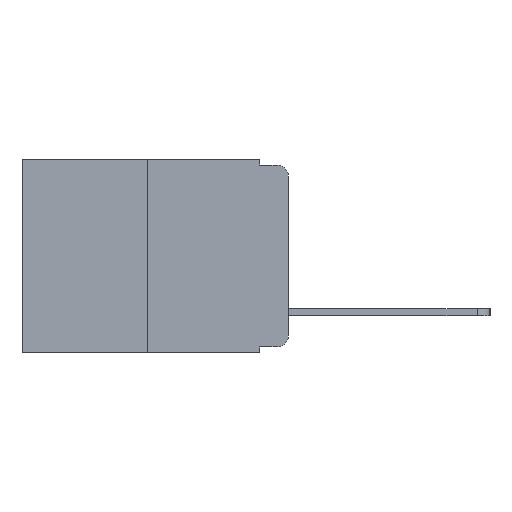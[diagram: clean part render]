
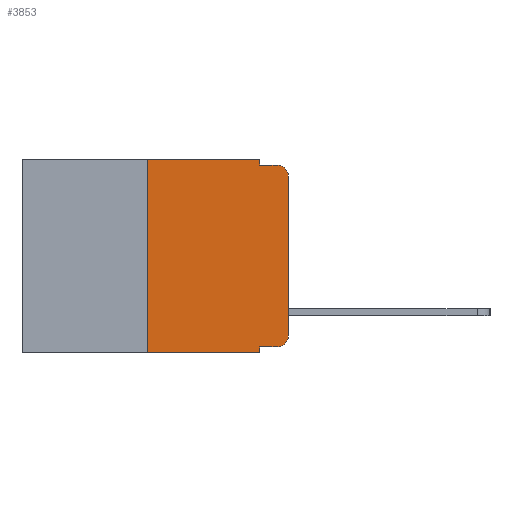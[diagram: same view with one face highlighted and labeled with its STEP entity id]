
A CAD part, left-side view. The second image highlights one B-rep face of the part: STEP entity #3853.
In plain terms, the highlighted planar face has unit normal (-1, 0, 0).
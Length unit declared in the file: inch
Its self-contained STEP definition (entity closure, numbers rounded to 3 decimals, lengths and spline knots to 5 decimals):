
#44 = VECTOR ( 'NONE', #3785, 39.37008 ) ;
#149 = EDGE_CURVE ( 'NONE', #6712, #3612, #3494, .T. ) ;
#217 = EDGE_CURVE ( 'NONE', #7142, #13199, #8737, .T. ) ;
#274 = DIRECTION ( 'NONE',  ( 0., 0., -1. ) ) ;
#323 = EDGE_CURVE ( 'NONE', #13199, #2902, #4007, .T. ) ;
#781 = EDGE_CURVE ( 'NONE', #3612, #11555, #12100, .T. ) ;
#903 = ORIENTED_EDGE ( 'NONE', *, *, #1077, .F. ) ;
#914 = ORIENTED_EDGE ( 'NONE', *, *, #323, .T. ) ;
#958 = VECTOR ( 'NONE', #3587, 39.37008 ) ;
#1077 = EDGE_CURVE ( 'NONE', #7542, #7985, #8708, .T. ) ;
#1640 = VECTOR ( 'NONE', #6236, 39.37008 ) ;
#1659 = CARTESIAN_POINT ( 'NONE',  ( 0., 0.473, 0. ) ) ;
#1735 = VECTOR ( 'NONE', #9234, 39.37008 ) ;
#1917 = CARTESIAN_POINT ( 'NONE',  ( 0., 0.051, 0. ) ) ;
#2018 = PLANE ( 'NONE',  #10224 ) ;
#2061 = LINE ( 'NONE', #8143, #1735 ) ;
#2401 = DIRECTION ( 'NONE',  ( 0., 0., -1. ) ) ;
#2510 = DIRECTION ( 'NONE',  ( 0., 0., 1. ) ) ;
#2614 = FACE_OUTER_BOUND ( 'NONE', #3389, .T. ) ;
#2816 = CARTESIAN_POINT ( 'NONE',  ( 0., 0.25, 0. ) ) ;
#2818 = ORIENTED_EDGE ( 'NONE', *, *, #13155, .T. ) ;
#2899 = LINE ( 'NONE', #3506, #44 ) ;
#2902 = VERTEX_POINT ( 'NONE', #8677 ) ;
#3178 = CARTESIAN_POINT ( 'NONE',  ( 0., 0., 0. ) ) ;
#3389 = EDGE_LOOP ( 'NONE', ( #914, #2818, #11220, #7146, #13559, #10040, #9692, #903, #11549, #11213 ) ) ;
#3494 = LINE ( 'NONE', #6247, #958 ) ;
#3506 = CARTESIAN_POINT ( 'NONE',  ( 0., 0.473, -0.343 ) ) ;
#3587 = DIRECTION ( 'NONE',  ( 0., -1., 0. ) ) ;
#3612 = VERTEX_POINT ( 'NONE', #1917 ) ;
#3785 = DIRECTION ( 'NONE',  ( 0., -1., 0. ) ) ;
#3853 = ADVANCED_FACE ( 'NONE', ( #2614 ), #2018, .F. ) ;
#4007 = LINE ( 'NONE', #3178, #6672 ) ;
#4247 = CARTESIAN_POINT ( 'NONE',  ( 0., 0.051, 0. ) ) ;
#4394 = CARTESIAN_POINT ( 'NONE',  ( 0., 0.02, -0.01 ) ) ;
#4531 = LINE ( 'NONE', #12755, #1640 ) ;
#4721 = VERTEX_POINT ( 'NONE', #4394 ) ;
#5184 = AXIS2_PLACEMENT_3D ( 'NONE', #13366, #6913, #274 ) ;
#5213 = EDGE_CURVE ( 'NONE', #13657, #7985, #2899, .T. ) ;
#5499 = LINE ( 'NONE', #10688, #11020 ) ;
#6114 = EDGE_CURVE ( 'NONE', #7542, #7142, #5499, .T. ) ;
#6236 = DIRECTION ( 'NONE',  ( 0., -1., 0. ) ) ;
#6247 = CARTESIAN_POINT ( 'NONE',  ( 0., 0.473, 0. ) ) ;
#6658 = CARTESIAN_POINT ( 'NONE',  ( 0., 0.051, -0.01 ) ) ;
#6672 = VECTOR ( 'NONE', #2510, 39.37008 ) ;
#6712 = VERTEX_POINT ( 'NONE', #2816 ) ;
#6913 = DIRECTION ( 'NONE',  ( -1., 0., 0. ) ) ;
#6965 = CARTESIAN_POINT ( 'NONE',  ( 0., 0.02, -0.333 ) ) ;
#7142 = VERTEX_POINT ( 'NONE', #6965 ) ;
#7146 = ORIENTED_EDGE ( 'NONE', *, *, #781, .F. ) ;
#7542 = VERTEX_POINT ( 'NONE', #7673 ) ;
#7673 = CARTESIAN_POINT ( 'NONE',  ( 0., 0.051, -0.333 ) ) ;
#7695 = VECTOR ( 'NONE', #9508, 39.37008 ) ;
#7764 = CARTESIAN_POINT ( 'NONE',  ( 0., 0.25, -0.343 ) ) ;
#7985 = VERTEX_POINT ( 'NONE', #8333 ) ;
#8072 = CARTESIAN_POINT ( 'NONE',  ( 0., 0., -0.313 ) ) ;
#8143 = CARTESIAN_POINT ( 'NONE',  ( 0., 0.25, 0. ) ) ;
#8333 = CARTESIAN_POINT ( 'NONE',  ( 0., 0.051, -0.343 ) ) ;
#8677 = CARTESIAN_POINT ( 'NONE',  ( 0., 0., -0.03 ) ) ;
#8708 = LINE ( 'NONE', #13392, #7695 ) ;
#8737 = CIRCLE ( 'NONE', #11533, 0.02 ) ;
#9234 = DIRECTION ( 'NONE',  ( 0., 0., 1. ) ) ;
#9508 = DIRECTION ( 'NONE',  ( 0., 0., -1. ) ) ;
#9692 = ORIENTED_EDGE ( 'NONE', *, *, #5213, .T. ) ;
#10040 = ORIENTED_EDGE ( 'NONE', *, *, #12607, .F. ) ;
#10224 = AXIS2_PLACEMENT_3D ( 'NONE', #1659, #11684, #11647 ) ;
#10688 = CARTESIAN_POINT ( 'NONE',  ( 0., 0.051, -0.333 ) ) ;
#11020 = VECTOR ( 'NONE', #11771, 39.37008 ) ;
#11213 = ORIENTED_EDGE ( 'NONE', *, *, #217, .T. ) ;
#11220 = ORIENTED_EDGE ( 'NONE', *, *, #13425, .F. ) ;
#11357 = CIRCLE ( 'NONE', #5184, 0.02 ) ;
#11533 = AXIS2_PLACEMENT_3D ( 'NONE', #12991, #13005, #12019 ) ;
#11549 = ORIENTED_EDGE ( 'NONE', *, *, #6114, .T. ) ;
#11555 = VERTEX_POINT ( 'NONE', #6658 ) ;
#11647 = DIRECTION ( 'NONE',  ( 0., 0., -1. ) ) ;
#11684 = DIRECTION ( 'NONE',  ( 1., 0., 0. ) ) ;
#11760 = VECTOR ( 'NONE', #2401, 39.37008 ) ;
#11771 = DIRECTION ( 'NONE',  ( 0., -1., 0. ) ) ;
#12019 = DIRECTION ( 'NONE',  ( 0., 0., -1. ) ) ;
#12100 = LINE ( 'NONE', #4247, #11760 ) ;
#12607 = EDGE_CURVE ( 'NONE', #13657, #6712, #2061, .T. ) ;
#12755 = CARTESIAN_POINT ( 'NONE',  ( 0., 0.051, -0.01 ) ) ;
#12991 = CARTESIAN_POINT ( 'NONE',  ( 0., 0.02, -0.313 ) ) ;
#13005 = DIRECTION ( 'NONE',  ( -1., 0., 0. ) ) ;
#13155 = EDGE_CURVE ( 'NONE', #2902, #4721, #11357, .T. ) ;
#13199 = VERTEX_POINT ( 'NONE', #8072 ) ;
#13366 = CARTESIAN_POINT ( 'NONE',  ( 0., 0.02, -0.03 ) ) ;
#13392 = CARTESIAN_POINT ( 'NONE',  ( 0., 0.051, 0. ) ) ;
#13425 = EDGE_CURVE ( 'NONE', #11555, #4721, #4531, .T. ) ;
#13559 = ORIENTED_EDGE ( 'NONE', *, *, #149, .F. ) ;
#13657 = VERTEX_POINT ( 'NONE', #7764 ) ;
